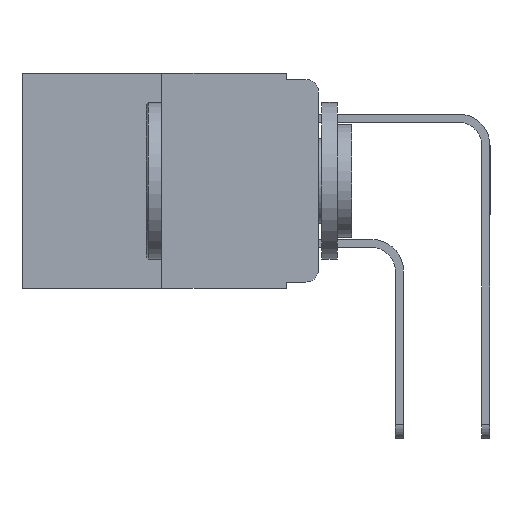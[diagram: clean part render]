
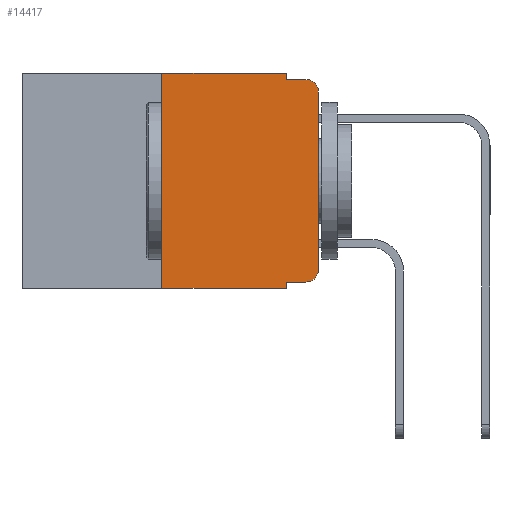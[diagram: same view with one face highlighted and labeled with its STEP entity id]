
A CAD part, left-side view. The second image highlights one B-rep face of the part: STEP entity #14417.
In plain terms, the highlighted planar face has unit normal (-1, 0, 0).
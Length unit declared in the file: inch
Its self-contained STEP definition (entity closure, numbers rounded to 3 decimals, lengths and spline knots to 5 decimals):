
#32 = AXIS2_PLACEMENT_3D ( 'NONE', #7135, #2036, #1963 ) ;
#349 = CARTESIAN_POINT ( 'NONE',  ( 0., 0.051, -0.01 ) ) ;
#658 = DIRECTION ( 'NONE',  ( 0., 0., 1. ) ) ;
#712 = EDGE_CURVE ( 'NONE', #6422, #17536, #12601, .T. ) ;
#724 = LINE ( 'NONE', #5851, #15750 ) ;
#859 = DIRECTION ( 'NONE',  ( 0., 0., -1. ) ) ;
#1351 = AXIS2_PLACEMENT_3D ( 'NONE', #7223, #16984, #8693 ) ;
#1963 = DIRECTION ( 'NONE',  ( 0., 0., -1. ) ) ;
#2036 = DIRECTION ( 'NONE',  ( -1., 0., 0. ) ) ;
#2292 = AXIS2_PLACEMENT_3D ( 'NONE', #12631, #9908, #859 ) ;
#2441 = ORIENTED_EDGE ( 'NONE', *, *, #15716, .F. ) ;
#2476 = VERTEX_POINT ( 'NONE', #15531 ) ;
#2648 = VERTEX_POINT ( 'NONE', #6194 ) ;
#2903 = VECTOR ( 'NONE', #12688, 39.37008 ) ;
#2904 = EDGE_CURVE ( 'NONE', #12886, #6422, #3971, .T. ) ;
#2946 = EDGE_LOOP ( 'NONE', ( #3925, #12035, #16767, #2441, #4405, #5327, #16782, #10329, #5345, #6523 ) ) ;
#3572 = VECTOR ( 'NONE', #10981, 39.37008 ) ;
#3925 = ORIENTED_EDGE ( 'NONE', *, *, #2904, .T. ) ;
#3971 = LINE ( 'NONE', #16605, #7410 ) ;
#4405 = ORIENTED_EDGE ( 'NONE', *, *, #4840, .F. ) ;
#4434 = DIRECTION ( 'NONE',  ( 0., 0., -1. ) ) ;
#4624 = VERTEX_POINT ( 'NONE', #349 ) ;
#4840 = EDGE_CURVE ( 'NONE', #6104, #2648, #10696, .T. ) ;
#5298 = CIRCLE ( 'NONE', #1351, 0.02 ) ;
#5316 = VECTOR ( 'NONE', #15658, 39.37008 ) ;
#5327 = ORIENTED_EDGE ( 'NONE', *, *, #14800, .F. ) ;
#5345 = ORIENTED_EDGE ( 'NONE', *, *, #12962, .T. ) ;
#5473 = CARTESIAN_POINT ( 'NONE',  ( 0., 0.25, 0. ) ) ;
#5851 = CARTESIAN_POINT ( 'NONE',  ( 0., 0.051, 0. ) ) ;
#6104 = VERTEX_POINT ( 'NONE', #5473 ) ;
#6194 = CARTESIAN_POINT ( 'NONE',  ( 0., 0.051, 0. ) ) ;
#6422 = VERTEX_POINT ( 'NONE', #8915 ) ;
#6523 = ORIENTED_EDGE ( 'NONE', *, *, #12041, .T. ) ;
#7135 = CARTESIAN_POINT ( 'NONE',  ( 0., 0.02, -0.03 ) ) ;
#7223 = CARTESIAN_POINT ( 'NONE',  ( 0., 0.02, -0.313 ) ) ;
#7410 = VECTOR ( 'NONE', #658, 39.37008 ) ;
#8125 = VECTOR ( 'NONE', #13433, 39.37008 ) ;
#8514 = EDGE_CURVE ( 'NONE', #16318, #8628, #16224, .T. ) ;
#8628 = VERTEX_POINT ( 'NONE', #12760 ) ;
#8693 = DIRECTION ( 'NONE',  ( 0., 0., -1. ) ) ;
#8783 = VECTOR ( 'NONE', #17524, 39.37008 ) ;
#8851 = VECTOR ( 'NONE', #13909, 39.37008 ) ;
#8915 = CARTESIAN_POINT ( 'NONE',  ( 0., 0., -0.03 ) ) ;
#9203 = CARTESIAN_POINT ( 'NONE',  ( 0., 0.25, 0. ) ) ;
#9908 = DIRECTION ( 'NONE',  ( 1., 0., 0. ) ) ;
#9915 = CARTESIAN_POINT ( 'NONE',  ( 0., 0.473, 0. ) ) ;
#10329 = ORIENTED_EDGE ( 'NONE', *, *, #13883, .F. ) ;
#10696 = LINE ( 'NONE', #9915, #2903 ) ;
#10981 = DIRECTION ( 'NONE',  ( 0., -1., 0. ) ) ;
#11717 = LINE ( 'NONE', #17803, #3572 ) ;
#12035 = ORIENTED_EDGE ( 'NONE', *, *, #712, .T. ) ;
#12041 = EDGE_CURVE ( 'NONE', #2476, #12886, #5298, .T. ) ;
#12043 = CARTESIAN_POINT ( 'NONE',  ( 0., 0.051, -0.01 ) ) ;
#12529 = CARTESIAN_POINT ( 'NONE',  ( 0., 0.473, -0.343 ) ) ;
#12601 = CIRCLE ( 'NONE', #32, 0.02 ) ;
#12631 = CARTESIAN_POINT ( 'NONE',  ( 0., 0.473, 0. ) ) ;
#12688 = DIRECTION ( 'NONE',  ( 0., -1., 0. ) ) ;
#12760 = CARTESIAN_POINT ( 'NONE',  ( 0., 0.051, -0.343 ) ) ;
#12886 = VERTEX_POINT ( 'NONE', #14958 ) ;
#12895 = LINE ( 'NONE', #14275, #5316 ) ;
#12962 = EDGE_CURVE ( 'NONE', #15622, #2476, #11717, .T. ) ;
#13433 = DIRECTION ( 'NONE',  ( 0., -1., 0. ) ) ;
#13883 = EDGE_CURVE ( 'NONE', #15622, #8628, #724, .T. ) ;
#13909 = DIRECTION ( 'NONE',  ( 0., -1., 0. ) ) ;
#14275 = CARTESIAN_POINT ( 'NONE',  ( 0., 0.051, 0. ) ) ;
#14417 = ADVANCED_FACE ( 'NONE', ( #18498 ), #15319, .F. ) ;
#14800 = EDGE_CURVE ( 'NONE', #16318, #6104, #16152, .T. ) ;
#14958 = CARTESIAN_POINT ( 'NONE',  ( 0., 0., -0.313 ) ) ;
#15319 = PLANE ( 'NONE',  #2292 ) ;
#15531 = CARTESIAN_POINT ( 'NONE',  ( 0., 0.02, -0.333 ) ) ;
#15537 = LINE ( 'NONE', #12043, #8125 ) ;
#15622 = VERTEX_POINT ( 'NONE', #16561 ) ;
#15658 = DIRECTION ( 'NONE',  ( 0., 0., -1. ) ) ;
#15716 = EDGE_CURVE ( 'NONE', #2648, #4624, #12895, .T. ) ;
#15750 = VECTOR ( 'NONE', #4434, 39.37008 ) ;
#16152 = LINE ( 'NONE', #9203, #8783 ) ;
#16224 = LINE ( 'NONE', #12529, #8851 ) ;
#16318 = VERTEX_POINT ( 'NONE', #16899 ) ;
#16561 = CARTESIAN_POINT ( 'NONE',  ( 0., 0.051, -0.333 ) ) ;
#16605 = CARTESIAN_POINT ( 'NONE',  ( 0., 0., 0. ) ) ;
#16767 = ORIENTED_EDGE ( 'NONE', *, *, #18454, .F. ) ;
#16782 = ORIENTED_EDGE ( 'NONE', *, *, #8514, .T. ) ;
#16899 = CARTESIAN_POINT ( 'NONE',  ( 0., 0.25, -0.343 ) ) ;
#16977 = CARTESIAN_POINT ( 'NONE',  ( 0., 0.02, -0.01 ) ) ;
#16984 = DIRECTION ( 'NONE',  ( -1., 0., 0. ) ) ;
#17524 = DIRECTION ( 'NONE',  ( 0., 0., 1. ) ) ;
#17536 = VERTEX_POINT ( 'NONE', #16977 ) ;
#17803 = CARTESIAN_POINT ( 'NONE',  ( 0., 0.051, -0.333 ) ) ;
#18454 = EDGE_CURVE ( 'NONE', #4624, #17536, #15537, .T. ) ;
#18498 = FACE_OUTER_BOUND ( 'NONE', #2946, .T. ) ;
